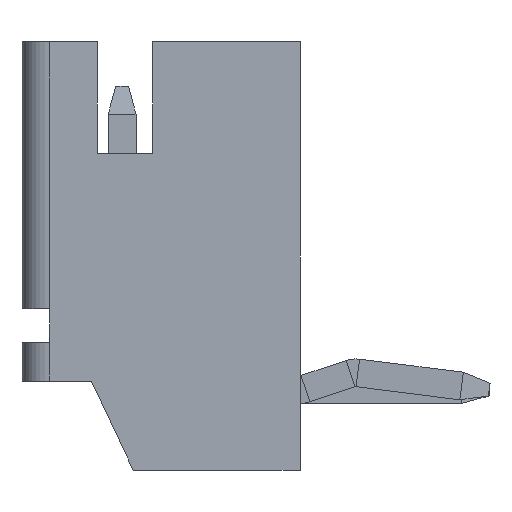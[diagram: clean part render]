
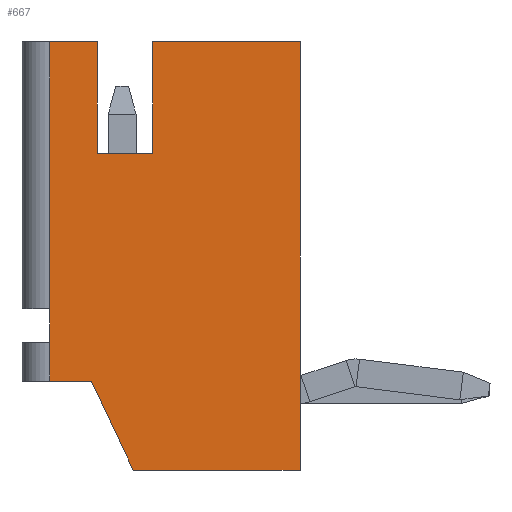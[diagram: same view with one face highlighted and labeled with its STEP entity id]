
A CAD part, left-side view. The second image highlights one B-rep face of the part: STEP entity #667.
In plain terms, the highlighted planar face has unit normal (-1, 0, 0).
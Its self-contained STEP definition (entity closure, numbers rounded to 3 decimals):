
#44 = EDGE_CURVE ( 'NONE', #5396, #4325, #2386, .T. ) ;
#73 = CARTESIAN_POINT ( 'NONE',  ( -2., -0.55, 6.1 ) ) ;
#101 = VECTOR ( 'NONE', #1786, 1000. ) ;
#161 = VERTEX_POINT ( 'NONE', #668 ) ;
#206 = VERTEX_POINT ( 'NONE', #3997 ) ;
#259 = EDGE_CURVE ( 'NONE', #206, #2435, #4048, .T. ) ;
#348 = CARTESIAN_POINT ( 'NONE',  ( -2., 1.3, 0. ) ) ;
#365 = ORIENTED_EDGE ( 'NONE', *, *, #44, .T. ) ;
#392 = CARTESIAN_POINT ( 'NONE',  ( -2., 0.45, 4.1 ) ) ;
#458 = DIRECTION ( 'NONE',  ( 0., 0., -1. ) ) ;
#522 = EDGE_LOOP ( 'NONE', ( #746, #2165, #5695, #3580, #5249, #3868, #4990, #1754, #5319, #4827, #365, #1822 ) ) ;
#558 = CARTESIAN_POINT ( 'NONE',  ( -2., 1.3, 0.7 ) ) ;
#667 = ADVANCED_FACE ( 'NONE', ( #5892 ), #4889, .T. ) ;
#668 = CARTESIAN_POINT ( 'NONE',  ( -2., -0.2, -1.6 ) ) ;
#741 = DIRECTION ( 'NONE',  ( 0., 0., -1. ) ) ;
#746 = ORIENTED_EDGE ( 'NONE', *, *, #2003, .T. ) ;
#858 = LINE ( 'NONE', #2591, #5449 ) ;
#1004 = CARTESIAN_POINT ( 'NONE',  ( -2., -0.2, -1.6 ) ) ;
#1069 = VECTOR ( 'NONE', #1757, 1000. ) ;
#1120 = CARTESIAN_POINT ( 'NONE',  ( -2., 0., 0. ) ) ;
#1447 = EDGE_CURVE ( 'NONE', #2435, #4151, #5435, .T. ) ;
#1587 = LINE ( 'NONE', #1004, #4370 ) ;
#1712 = EDGE_CURVE ( 'NONE', #5462, #5855, #1783, .T. ) ;
#1741 = EDGE_CURVE ( 'NONE', #5855, #5396, #5882, .T. ) ;
#1754 = ORIENTED_EDGE ( 'NONE', *, *, #2773, .T. ) ;
#1757 = DIRECTION ( 'NONE',  ( 0., 1., 0. ) ) ;
#1780 = EDGE_CURVE ( 'NONE', #3966, #1901, #3041, .T. ) ;
#1783 = LINE ( 'NONE', #2457, #2750 ) ;
#1786 = DIRECTION ( 'NONE',  ( 0., -1., 0. ) ) ;
#1822 = ORIENTED_EDGE ( 'NONE', *, *, #2194, .T. ) ;
#1901 = VERTEX_POINT ( 'NONE', #3940 ) ;
#2003 = EDGE_CURVE ( 'NONE', #3865, #6044, #3244, .T. ) ;
#2015 = VECTOR ( 'NONE', #741, 1000. ) ;
#2021 = DIRECTION ( 'NONE',  ( 0., -1., 0. ) ) ;
#2053 = CARTESIAN_POINT ( 'NONE',  ( -2., 1.3, 6.1 ) ) ;
#2063 = DIRECTION ( 'NONE',  ( -1., 0., 0. ) ) ;
#2165 = ORIENTED_EDGE ( 'NONE', *, *, #3735, .T. ) ;
#2194 = EDGE_CURVE ( 'NONE', #4325, #3865, #6019, .T. ) ;
#2313 = CARTESIAN_POINT ( 'NONE',  ( -2., 1.3, 0. ) ) ;
#2386 = LINE ( 'NONE', #3302, #2680 ) ;
#2403 = LINE ( 'NONE', #4602, #101 ) ;
#2435 = VERTEX_POINT ( 'NONE', #3418 ) ;
#2457 = CARTESIAN_POINT ( 'NONE',  ( -2., 0.45, 4.1 ) ) ;
#2591 = CARTESIAN_POINT ( 'NONE',  ( -2., 1.3, 0. ) ) ;
#2627 = CARTESIAN_POINT ( 'NONE',  ( -2., -3.2, 6.1 ) ) ;
#2650 = CARTESIAN_POINT ( 'NONE',  ( -2., 1.3, 1.3 ) ) ;
#2680 = VECTOR ( 'NONE', #4780, 1000. ) ;
#2692 = CARTESIAN_POINT ( 'NONE',  ( -2., -0.55, 4.1 ) ) ;
#2750 = VECTOR ( 'NONE', #5633, 1000. ) ;
#2773 = EDGE_CURVE ( 'NONE', #4151, #5462, #3599, .T. ) ;
#2816 = VECTOR ( 'NONE', #3102, 1000. ) ;
#2887 = CARTESIAN_POINT ( 'NONE',  ( -2., -0.55, 6.1 ) ) ;
#2906 = DIRECTION ( 'NONE',  ( 0., -0.424, -0.905 ) ) ;
#3041 = LINE ( 'NONE', #3487, #6023 ) ;
#3102 = DIRECTION ( 'NONE',  ( 0., 0., 1. ) ) ;
#3244 = LINE ( 'NONE', #2650, #2015 ) ;
#3291 = DIRECTION ( 'NONE',  ( 0., 0., 1. ) ) ;
#3302 = CARTESIAN_POINT ( 'NONE',  ( -2., 1.8, 6.1 ) ) ;
#3418 = CARTESIAN_POINT ( 'NONE',  ( -2., -3.2, 6.1 ) ) ;
#3487 = CARTESIAN_POINT ( 'NONE',  ( -2., 1.8, 0. ) ) ;
#3535 = VECTOR ( 'NONE', #4231, 1000. ) ;
#3580 = ORIENTED_EDGE ( 'NONE', *, *, #4214, .T. ) ;
#3599 = LINE ( 'NONE', #73, #3535 ) ;
#3613 = VECTOR ( 'NONE', #458, 1000. ) ;
#3735 = EDGE_CURVE ( 'NONE', #6044, #3966, #858, .T. ) ;
#3865 = VERTEX_POINT ( 'NONE', #5226 ) ;
#3868 = ORIENTED_EDGE ( 'NONE', *, *, #259, .T. ) ;
#3940 = CARTESIAN_POINT ( 'NONE',  ( -2., 0.55, 0. ) ) ;
#3966 = VERTEX_POINT ( 'NONE', #2313 ) ;
#3997 = CARTESIAN_POINT ( 'NONE',  ( -2., -3.2, -1.6 ) ) ;
#4048 = LINE ( 'NONE', #2627, #2816 ) ;
#4151 = VERTEX_POINT ( 'NONE', #2887 ) ;
#4214 = EDGE_CURVE ( 'NONE', #1901, #161, #1587, .T. ) ;
#4231 = DIRECTION ( 'NONE',  ( 0., 0., -1. ) ) ;
#4325 = VERTEX_POINT ( 'NONE', #2053 ) ;
#4351 = VECTOR ( 'NONE', #3291, 1000. ) ;
#4370 = VECTOR ( 'NONE', #2906, 1000. ) ;
#4497 = DIRECTION ( 'NONE',  ( 0., 0., -1. ) ) ;
#4516 = AXIS2_PLACEMENT_3D ( 'NONE', #1120, #2063, #2021 ) ;
#4602 = CARTESIAN_POINT ( 'NONE',  ( -2., -3.2, -1.6 ) ) ;
#4734 = EDGE_CURVE ( 'NONE', #161, #206, #2403, .T. ) ;
#4780 = DIRECTION ( 'NONE',  ( 0., 1., 0. ) ) ;
#4827 = ORIENTED_EDGE ( 'NONE', *, *, #1741, .T. ) ;
#4889 = PLANE ( 'NONE',  #4516 ) ;
#4990 = ORIENTED_EDGE ( 'NONE', *, *, #1447, .T. ) ;
#5091 = CARTESIAN_POINT ( 'NONE',  ( -2., -0.55, 6.1 ) ) ;
#5226 = CARTESIAN_POINT ( 'NONE',  ( -2., 1.3, 1.3 ) ) ;
#5249 = ORIENTED_EDGE ( 'NONE', *, *, #4734, .T. ) ;
#5319 = ORIENTED_EDGE ( 'NONE', *, *, #1712, .T. ) ;
#5396 = VERTEX_POINT ( 'NONE', #5516 ) ;
#5435 = LINE ( 'NONE', #5091, #1069 ) ;
#5449 = VECTOR ( 'NONE', #4497, 1000. ) ;
#5462 = VERTEX_POINT ( 'NONE', #2692 ) ;
#5516 = CARTESIAN_POINT ( 'NONE',  ( -2., 0.45, 6.1 ) ) ;
#5633 = DIRECTION ( 'NONE',  ( 0., 1., 0. ) ) ;
#5669 = CARTESIAN_POINT ( 'NONE',  ( -2., 0.45, 6.1 ) ) ;
#5695 = ORIENTED_EDGE ( 'NONE', *, *, #1780, .T. ) ;
#5760 = DIRECTION ( 'NONE',  ( 0., -1., 0. ) ) ;
#5855 = VERTEX_POINT ( 'NONE', #392 ) ;
#5882 = LINE ( 'NONE', #5669, #4351 ) ;
#5892 = FACE_OUTER_BOUND ( 'NONE', #522, .T. ) ;
#6019 = LINE ( 'NONE', #348, #3613 ) ;
#6023 = VECTOR ( 'NONE', #5760, 1000. ) ;
#6044 = VERTEX_POINT ( 'NONE', #558 ) ;
